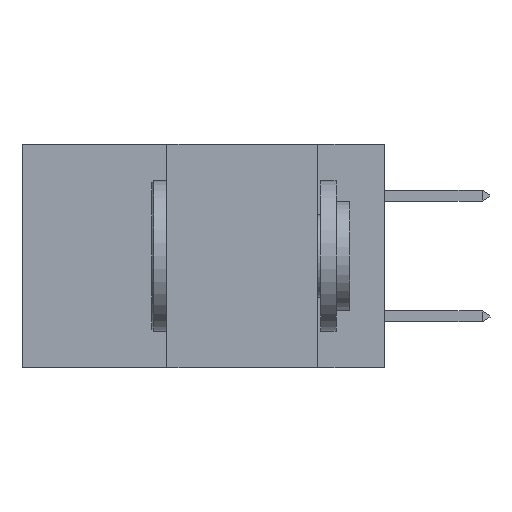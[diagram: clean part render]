
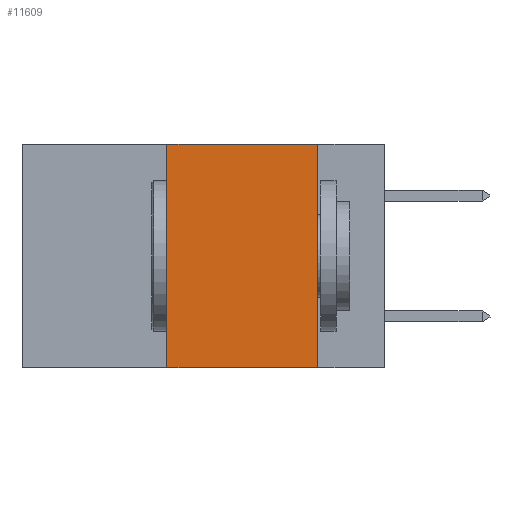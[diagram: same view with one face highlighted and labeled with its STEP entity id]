
A CAD part, left-side view. The second image highlights one B-rep face of the part: STEP entity #11609.
In plain terms, the highlighted planar face has unit normal (-1, 0, 0).
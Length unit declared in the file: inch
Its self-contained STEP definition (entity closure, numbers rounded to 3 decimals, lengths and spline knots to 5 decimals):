
#7 = VERTEX_POINT ( 'NONE', #10082 ) ;
#132 = DIRECTION ( 'NONE',  ( 1., 0., 0. ) ) ;
#596 = DIRECTION ( 'NONE',  ( 0., 0., 1. ) ) ;
#1426 = VECTOR ( 'NONE', #596, 39.37008 ) ;
#2366 = DIRECTION ( 'NONE',  ( 0., 0., -1. ) ) ;
#2544 = ORIENTED_EDGE ( 'NONE', *, *, #6726, .T. ) ;
#2612 = VERTEX_POINT ( 'NONE', #18488 ) ;
#3014 = LINE ( 'NONE', #19107, #13840 ) ;
#3491 = DIRECTION ( 'NONE',  ( 0., -1., 0. ) ) ;
#5420 = ORIENTED_EDGE ( 'NONE', *, *, #6808, .F. ) ;
#6125 = VERTEX_POINT ( 'NONE', #15391 ) ;
#6135 = DIRECTION ( 'NONE',  ( 0., -1., 0. ) ) ;
#6631 = LINE ( 'NONE', #22848, #1426 ) ;
#6726 = EDGE_CURVE ( 'NONE', #7, #6125, #3014, .T. ) ;
#6764 = EDGE_CURVE ( 'NONE', #2612, #6125, #21587, .T. ) ;
#6808 = EDGE_CURVE ( 'NONE', #7, #10438, #6631, .T. ) ;
#7528 = EDGE_CURVE ( 'NONE', #10438, #2612, #9011, .T. ) ;
#7603 = FACE_OUTER_BOUND ( 'NONE', #10730, .T. ) ;
#8466 = AXIS2_PLACEMENT_3D ( 'NONE', #15307, #132, #13598 ) ;
#9011 = LINE ( 'NONE', #14902, #18203 ) ;
#10082 = CARTESIAN_POINT ( 'NONE',  ( 0., 0.36, -0.37 ) ) ;
#10438 = VERTEX_POINT ( 'NONE', #14678 ) ;
#10730 = EDGE_LOOP ( 'NONE', ( #15184, #11044, #5420, #2544 ) ) ;
#11044 = ORIENTED_EDGE ( 'NONE', *, *, #7528, .F. ) ;
#11609 = ADVANCED_FACE ( 'NONE', ( #7603 ), #11758, .F. ) ;
#11758 = PLANE ( 'NONE',  #8466 ) ;
#13598 = DIRECTION ( 'NONE',  ( 0., 0., -1. ) ) ;
#13840 = VECTOR ( 'NONE', #6135, 39.37008 ) ;
#14678 = CARTESIAN_POINT ( 'NONE',  ( 0., 0.36, 0. ) ) ;
#14902 = CARTESIAN_POINT ( 'NONE',  ( 0., 0.6, 0. ) ) ;
#15184 = ORIENTED_EDGE ( 'NONE', *, *, #6764, .F. ) ;
#15307 = CARTESIAN_POINT ( 'NONE',  ( 0., 0.6, 0. ) ) ;
#15391 = CARTESIAN_POINT ( 'NONE',  ( 0., 0.11, -0.37 ) ) ;
#16352 = VECTOR ( 'NONE', #2366, 39.37008 ) ;
#18203 = VECTOR ( 'NONE', #3491, 39.37008 ) ;
#18488 = CARTESIAN_POINT ( 'NONE',  ( 0., 0.11, 0. ) ) ;
#19107 = CARTESIAN_POINT ( 'NONE',  ( 0., 0.6, -0.37 ) ) ;
#20938 = CARTESIAN_POINT ( 'NONE',  ( 0., 0.11, 0. ) ) ;
#21587 = LINE ( 'NONE', #20938, #16352 ) ;
#22848 = CARTESIAN_POINT ( 'NONE',  ( 0., 0.36, 0. ) ) ;
